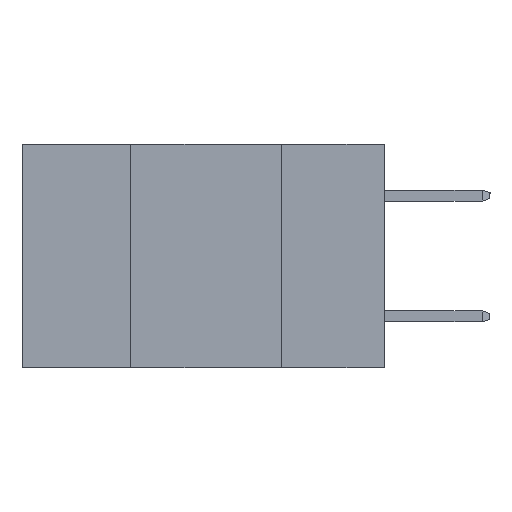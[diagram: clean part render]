
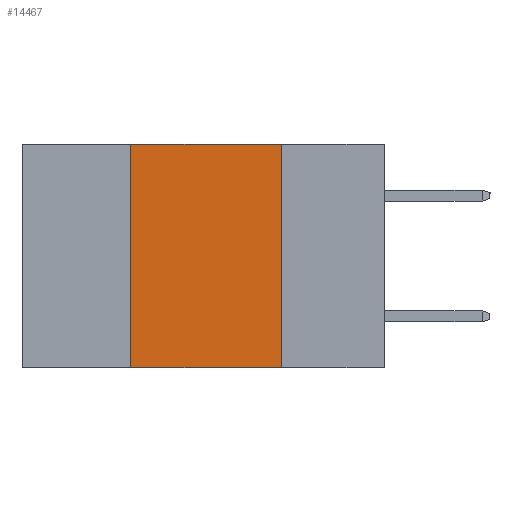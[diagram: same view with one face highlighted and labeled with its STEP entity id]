
A CAD part, left-side view. The second image highlights one B-rep face of the part: STEP entity #14467.
In plain terms, the highlighted planar face has unit normal (-1, 0, 0).
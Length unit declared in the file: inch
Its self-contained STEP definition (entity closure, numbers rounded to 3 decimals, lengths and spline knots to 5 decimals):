
#276 = DIRECTION ( 'NONE',  ( 0., 0., -1. ) ) ;
#422 = ORIENTED_EDGE ( 'NONE', *, *, #4037, .F. ) ;
#1239 = VERTEX_POINT ( 'NONE', #1665 ) ;
#1272 = VECTOR ( 'NONE', #12668, 39.37008 ) ;
#1665 = CARTESIAN_POINT ( 'NONE',  ( 0., 0.42, 0. ) ) ;
#1703 = LINE ( 'NONE', #6053, #10908 ) ;
#3884 = AXIS2_PLACEMENT_3D ( 'NONE', #10513, #11737, #9445 ) ;
#4037 = EDGE_CURVE ( 'NONE', #1239, #7596, #8090, .T. ) ;
#4647 = CARTESIAN_POINT ( 'NONE',  ( 0., 0.6, 0. ) ) ;
#5189 = EDGE_CURVE ( 'NONE', #8658, #1239, #8208, .T. ) ;
#5599 = CARTESIAN_POINT ( 'NONE',  ( 0., 0.17, 0. ) ) ;
#6053 = CARTESIAN_POINT ( 'NONE',  ( 0., 0.17, -0.37 ) ) ;
#6064 = FACE_OUTER_BOUND ( 'NONE', #14171, .T. ) ;
#7024 = CARTESIAN_POINT ( 'NONE',  ( 0., 0.6, -0.37 ) ) ;
#7060 = CARTESIAN_POINT ( 'NONE',  ( 0., 0.42, -0.37 ) ) ;
#7596 = VERTEX_POINT ( 'NONE', #5599 ) ;
#8090 = LINE ( 'NONE', #4647, #1272 ) ;
#8208 = LINE ( 'NONE', #7060, #10210 ) ;
#8658 = VERTEX_POINT ( 'NONE', #10763 ) ;
#8755 = ORIENTED_EDGE ( 'NONE', *, *, #14045, .T. ) ;
#9276 = CARTESIAN_POINT ( 'NONE',  ( 0., 0.17, -0.37 ) ) ;
#9445 = DIRECTION ( 'NONE',  ( 0., 0., -1. ) ) ;
#10210 = VECTOR ( 'NONE', #11573, 39.37008 ) ;
#10264 = ORIENTED_EDGE ( 'NONE', *, *, #10919, .F. ) ;
#10513 = CARTESIAN_POINT ( 'NONE',  ( 0., 0.6, 0. ) ) ;
#10741 = VERTEX_POINT ( 'NONE', #9276 ) ;
#10763 = CARTESIAN_POINT ( 'NONE',  ( 0., 0.42, -0.37 ) ) ;
#10908 = VECTOR ( 'NONE', #276, 39.37008 ) ;
#10919 = EDGE_CURVE ( 'NONE', #7596, #10741, #1703, .T. ) ;
#11573 = DIRECTION ( 'NONE',  ( 0., 0., 1. ) ) ;
#11723 = ORIENTED_EDGE ( 'NONE', *, *, #5189, .F. ) ;
#11737 = DIRECTION ( 'NONE',  ( 1., 0., 0. ) ) ;
#12523 = DIRECTION ( 'NONE',  ( 0., -1., 0. ) ) ;
#12668 = DIRECTION ( 'NONE',  ( 0., -1., 0. ) ) ;
#13640 = VECTOR ( 'NONE', #12523, 39.37008 ) ;
#13868 = PLANE ( 'NONE',  #3884 ) ;
#14045 = EDGE_CURVE ( 'NONE', #8658, #10741, #14065, .T. ) ;
#14065 = LINE ( 'NONE', #7024, #13640 ) ;
#14171 = EDGE_LOOP ( 'NONE', ( #10264, #422, #11723, #8755 ) ) ;
#14467 = ADVANCED_FACE ( 'NONE', ( #6064 ), #13868, .F. ) ;
